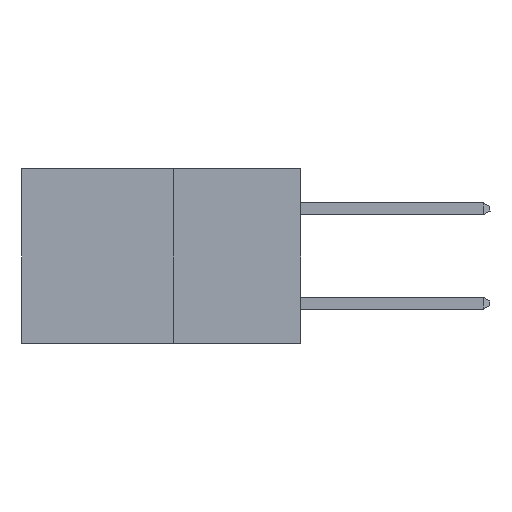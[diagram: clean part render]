
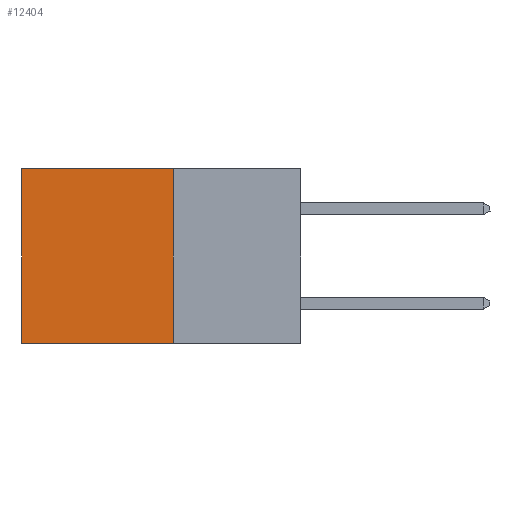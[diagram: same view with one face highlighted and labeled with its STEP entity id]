
A CAD part, left-side view. The second image highlights one B-rep face of the part: STEP entity #12404.
In plain terms, the highlighted planar face has unit normal (-1, 0, 0).
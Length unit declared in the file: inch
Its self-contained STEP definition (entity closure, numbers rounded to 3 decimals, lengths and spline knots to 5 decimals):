
#325 = CARTESIAN_POINT ( 'NONE',  ( 0.277, 0.27, 0. ) ) ;
#825 = CARTESIAN_POINT ( 'NONE',  ( 0.277, 0.27, -0.37 ) ) ;
#2679 = CARTESIAN_POINT ( 'NONE',  ( 0.277, 0.27, 0. ) ) ;
#3035 = VECTOR ( 'NONE', #18629, 39.37008 ) ;
#3668 = LINE ( 'NONE', #825, #20778 ) ;
#3694 = LINE ( 'NONE', #17605, #3035 ) ;
#3752 = AXIS2_PLACEMENT_3D ( 'NONE', #25668, #5346, #19864 ) ;
#3941 = EDGE_LOOP ( 'NONE', ( #22573, #19775, #7016, #14575 ) ) ;
#4277 = VERTEX_POINT ( 'NONE', #26130 ) ;
#5346 = DIRECTION ( 'NONE',  ( 1., 0., 0. ) ) ;
#5419 = EDGE_CURVE ( 'NONE', #17529, #7466, #3694, .T. ) ;
#7002 = DIRECTION ( 'NONE',  ( 0., 1., 0. ) ) ;
#7016 = ORIENTED_EDGE ( 'NONE', *, *, #5419, .F. ) ;
#7466 = VERTEX_POINT ( 'NONE', #16695 ) ;
#8980 = VECTOR ( 'NONE', #14082, 39.37008 ) ;
#9235 = FACE_OUTER_BOUND ( 'NONE', #3941, .T. ) ;
#11584 = CARTESIAN_POINT ( 'NONE',  ( 0.277, 0.59, 0. ) ) ;
#12073 = CARTESIAN_POINT ( 'NONE',  ( 0.277, 0.59, -0.37 ) ) ;
#12404 = ADVANCED_FACE ( 'NONE', ( #9235 ), #17708, .F. ) ;
#14082 = DIRECTION ( 'NONE',  ( 0., 0., -1. ) ) ;
#14575 = ORIENTED_EDGE ( 'NONE', *, *, #24038, .T. ) ;
#16695 = CARTESIAN_POINT ( 'NONE',  ( 0.277, 0.27, -0.37 ) ) ;
#17239 = EDGE_CURVE ( 'NONE', #21221, #4277, #24573, .T. ) ;
#17529 = VERTEX_POINT ( 'NONE', #325 ) ;
#17605 = CARTESIAN_POINT ( 'NONE',  ( 0.277, 0.27, -0.37 ) ) ;
#17708 = PLANE ( 'NONE',  #3752 ) ;
#18629 = DIRECTION ( 'NONE',  ( 0., 0., -1. ) ) ;
#19775 = ORIENTED_EDGE ( 'NONE', *, *, #22792, .F. ) ;
#19864 = DIRECTION ( 'NONE',  ( 0., 0., -1. ) ) ;
#19986 = VECTOR ( 'NONE', #23187, 39.37008 ) ;
#20597 = LINE ( 'NONE', #2679, #19986 ) ;
#20778 = VECTOR ( 'NONE', #7002, 39.37008 ) ;
#21221 = VERTEX_POINT ( 'NONE', #11584 ) ;
#22573 = ORIENTED_EDGE ( 'NONE', *, *, #17239, .T. ) ;
#22792 = EDGE_CURVE ( 'NONE', #7466, #4277, #3668, .T. ) ;
#23187 = DIRECTION ( 'NONE',  ( 0., 1., 0. ) ) ;
#24038 = EDGE_CURVE ( 'NONE', #17529, #21221, #20597, .T. ) ;
#24573 = LINE ( 'NONE', #12073, #8980 ) ;
#25668 = CARTESIAN_POINT ( 'NONE',  ( 0.277, 0.27, -0.37 ) ) ;
#26130 = CARTESIAN_POINT ( 'NONE',  ( 0.277, 0.59, -0.37 ) ) ;
